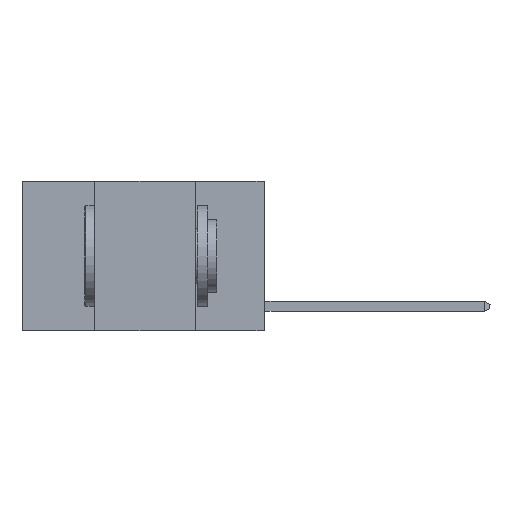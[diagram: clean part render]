
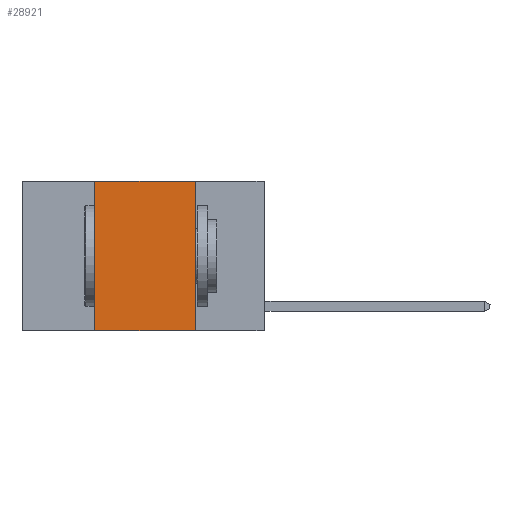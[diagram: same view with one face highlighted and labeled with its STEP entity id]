
A CAD part, left-side view. The second image highlights one B-rep face of the part: STEP entity #28921.
In plain terms, the highlighted planar face has unit normal (-1, 0, 0).
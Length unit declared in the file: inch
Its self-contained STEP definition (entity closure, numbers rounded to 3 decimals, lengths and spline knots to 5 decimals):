
#308 = LINE ( 'NONE', #20146, #23749 ) ;
#1096 = DIRECTION ( 'NONE',  ( 0., -1., 0. ) ) ;
#1715 = CARTESIAN_POINT ( 'NONE',  ( 0., 0.17, -0.37 ) ) ;
#3060 = EDGE_CURVE ( 'NONE', #21537, #3757, #17174, .T. ) ;
#3153 = VECTOR ( 'NONE', #1096, 39.37008 ) ;
#3686 = EDGE_CURVE ( 'NONE', #22844, #21537, #308, .T. ) ;
#3692 = ORIENTED_EDGE ( 'NONE', *, *, #17578, .T. ) ;
#3757 = VERTEX_POINT ( 'NONE', #1715 ) ;
#4046 = ORIENTED_EDGE ( 'NONE', *, *, #3060, .F. ) ;
#5412 = PLANE ( 'NONE',  #29475 ) ;
#7542 = CARTESIAN_POINT ( 'NONE',  ( 0., 0.42, 0. ) ) ;
#7720 = ORIENTED_EDGE ( 'NONE', *, *, #3686, .F. ) ;
#7762 = DIRECTION ( 'NONE',  ( 1., 0., 0. ) ) ;
#8439 = DIRECTION ( 'NONE',  ( 0., -1., 0. ) ) ;
#9396 = VECTOR ( 'NONE', #23116, 39.37008 ) ;
#10813 = LINE ( 'NONE', #12722, #3153 ) ;
#10921 = VECTOR ( 'NONE', #15637, 39.37008 ) ;
#12722 = CARTESIAN_POINT ( 'NONE',  ( 0., 0.6, -0.37 ) ) ;
#13340 = VERTEX_POINT ( 'NONE', #17494 ) ;
#14885 = LINE ( 'NONE', #20779, #9396 ) ;
#15637 = DIRECTION ( 'NONE',  ( 0., 0., -1. ) ) ;
#17168 = EDGE_CURVE ( 'NONE', #13340, #22844, #14885, .T. ) ;
#17174 = LINE ( 'NONE', #22616, #10921 ) ;
#17494 = CARTESIAN_POINT ( 'NONE',  ( 0., 0.42, -0.37 ) ) ;
#17578 = EDGE_CURVE ( 'NONE', #13340, #3757, #10813, .T. ) ;
#20146 = CARTESIAN_POINT ( 'NONE',  ( 0., 0.6, 0. ) ) ;
#20342 = FACE_OUTER_BOUND ( 'NONE', #25905, .T. ) ;
#20779 = CARTESIAN_POINT ( 'NONE',  ( 0., 0.42, 0. ) ) ;
#21537 = VERTEX_POINT ( 'NONE', #24033 ) ;
#21805 = CARTESIAN_POINT ( 'NONE',  ( 0., 0.6, 0. ) ) ;
#22616 = CARTESIAN_POINT ( 'NONE',  ( 0., 0.17, 0. ) ) ;
#22844 = VERTEX_POINT ( 'NONE', #7542 ) ;
#23116 = DIRECTION ( 'NONE',  ( 0., 0., 1. ) ) ;
#23749 = VECTOR ( 'NONE', #8439, 39.37008 ) ;
#24033 = CARTESIAN_POINT ( 'NONE',  ( 0., 0.17, 0. ) ) ;
#24145 = DIRECTION ( 'NONE',  ( 0., 0., -1. ) ) ;
#25905 = EDGE_LOOP ( 'NONE', ( #4046, #7720, #26386, #3692 ) ) ;
#26386 = ORIENTED_EDGE ( 'NONE', *, *, #17168, .F. ) ;
#28921 = ADVANCED_FACE ( 'NONE', ( #20342 ), #5412, .F. ) ;
#29475 = AXIS2_PLACEMENT_3D ( 'NONE', #21805, #7762, #24145 ) ;
